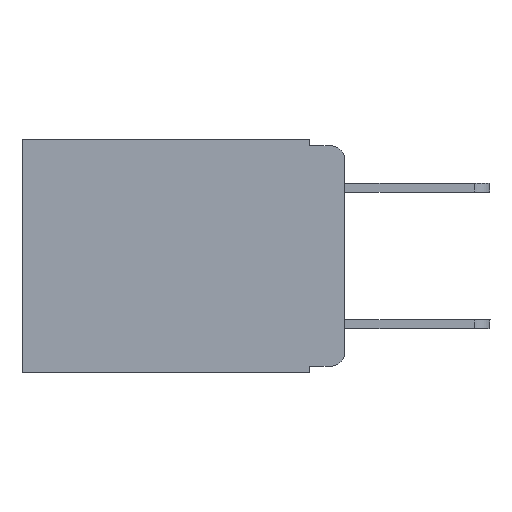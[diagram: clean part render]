
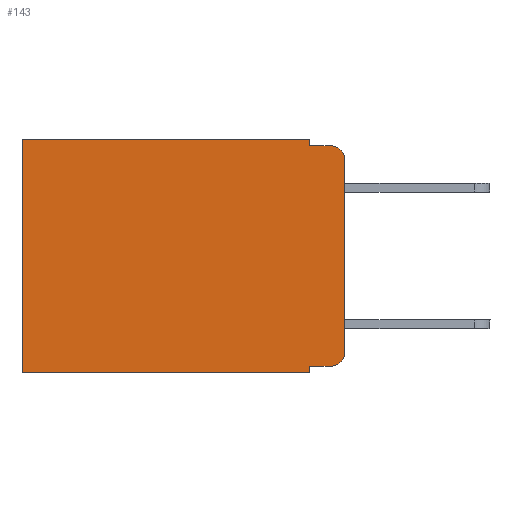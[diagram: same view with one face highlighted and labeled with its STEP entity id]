
A CAD part, left-side view. The second image highlights one B-rep face of the part: STEP entity #143.
In plain terms, the highlighted planar face has unit normal (-1, 0, 0).
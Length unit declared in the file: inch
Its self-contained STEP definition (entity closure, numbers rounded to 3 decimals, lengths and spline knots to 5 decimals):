
#33 = VERTEX_POINT ( 'NONE', #988 ) ;
#143 = ADVANCED_FACE ( 'NONE', ( #11187 ), #699, .F. ) ;
#487 = ORIENTED_EDGE ( 'NONE', *, *, #12742, .T. ) ;
#530 = CARTESIAN_POINT ( 'NONE',  ( 0.298, 0., 0. ) ) ;
#699 = PLANE ( 'NONE',  #9173 ) ;
#811 = CARTESIAN_POINT ( 'NONE',  ( 0.298, 0.02, -0.03 ) ) ;
#978 = LINE ( 'NONE', #1427, #16154 ) ;
#988 = CARTESIAN_POINT ( 'NONE',  ( 0.298, 0., -0.03 ) ) ;
#1113 = LINE ( 'NONE', #8055, #15606 ) ;
#1183 = LINE ( 'NONE', #4387, #14822 ) ;
#1300 = CARTESIAN_POINT ( 'NONE',  ( 0.298, 0., -0.343 ) ) ;
#1375 = EDGE_CURVE ( 'NONE', #7116, #10123, #978, .T. ) ;
#1427 = CARTESIAN_POINT ( 'NONE',  ( 0.298, 0.473, 0. ) ) ;
#1763 = LINE ( 'NONE', #530, #5654 ) ;
#1781 = EDGE_CURVE ( 'NONE', #33, #12541, #6381, .T. ) ;
#1877 = CARTESIAN_POINT ( 'NONE',  ( 0.298, 0., -0.313 ) ) ;
#1934 = CARTESIAN_POINT ( 'NONE',  ( 0.298, 0.051, 0. ) ) ;
#2156 = DIRECTION ( 'NONE',  ( 0., 0., -1. ) ) ;
#2339 = CARTESIAN_POINT ( 'NONE',  ( 0.298, 0.051, -0.333 ) ) ;
#2391 = DIRECTION ( 'NONE',  ( -1., 0., 0. ) ) ;
#2654 = VECTOR ( 'NONE', #15535, 39.37008 ) ;
#2884 = LINE ( 'NONE', #7291, #2654 ) ;
#3006 = CARTESIAN_POINT ( 'NONE',  ( 0.298, 0.02, -0.01 ) ) ;
#3070 = CARTESIAN_POINT ( 'NONE',  ( 0.298, 0.473, 0. ) ) ;
#3205 = LINE ( 'NONE', #7693, #15541 ) ;
#3398 = DIRECTION ( 'NONE',  ( -1., 0., 0. ) ) ;
#3602 = CIRCLE ( 'NONE', #17413, 0.02 ) ;
#3733 = EDGE_CURVE ( 'NONE', #12563, #12300, #2884, .T. ) ;
#3785 = CARTESIAN_POINT ( 'NONE',  ( 0.298, 0.02, -0.333 ) ) ;
#4387 = CARTESIAN_POINT ( 'NONE',  ( 0.298, 0.051, -0.333 ) ) ;
#4423 = EDGE_LOOP ( 'NONE', ( #15699, #9035, #10296, #15743, #487, #11450, #8967, #17879, #5829, #17066 ) ) ;
#4479 = EDGE_CURVE ( 'NONE', #12300, #10123, #14312, .T. ) ;
#4871 = CARTESIAN_POINT ( 'NONE',  ( 0.298, 0., 0. ) ) ;
#5654 = VECTOR ( 'NONE', #8736, 39.37008 ) ;
#5659 = CARTESIAN_POINT ( 'NONE',  ( 0.298, 0.051, -0.01 ) ) ;
#5804 = VERTEX_POINT ( 'NONE', #16118 ) ;
#5829 = ORIENTED_EDGE ( 'NONE', *, *, #7217, .T. ) ;
#6247 = DIRECTION ( 'NONE',  ( 1., 0., 0. ) ) ;
#6308 = VECTOR ( 'NONE', #10950, 39.37008 ) ;
#6381 = CIRCLE ( 'NONE', #12147, 0.02 ) ;
#6781 = VERTEX_POINT ( 'NONE', #1877 ) ;
#7116 = VERTEX_POINT ( 'NONE', #3070 ) ;
#7217 = EDGE_CURVE ( 'NONE', #12563, #13384, #1183, .T. ) ;
#7291 = CARTESIAN_POINT ( 'NONE',  ( 0.298, 0.051, 0. ) ) ;
#7483 = DIRECTION ( 'NONE',  ( 0., 0., -1. ) ) ;
#7693 = CARTESIAN_POINT ( 'NONE',  ( 0.298, 0., 0. ) ) ;
#8055 = CARTESIAN_POINT ( 'NONE',  ( 0.298, 0.051, 0. ) ) ;
#8473 = DIRECTION ( 'NONE',  ( 0., -1., 0. ) ) ;
#8688 = CARTESIAN_POINT ( 'NONE',  ( 0.298, 0.02, -0.313 ) ) ;
#8736 = DIRECTION ( 'NONE',  ( 0., 1., 0. ) ) ;
#8967 = ORIENTED_EDGE ( 'NONE', *, *, #4479, .F. ) ;
#9035 = ORIENTED_EDGE ( 'NONE', *, *, #1781, .T. ) ;
#9173 = AXIS2_PLACEMENT_3D ( 'NONE', #4871, #6247, #11904 ) ;
#9811 = CARTESIAN_POINT ( 'NONE',  ( 0.298, 0.473, -0.343 ) ) ;
#10123 = VERTEX_POINT ( 'NONE', #9811 ) ;
#10296 = ORIENTED_EDGE ( 'NONE', *, *, #13130, .F. ) ;
#10950 = DIRECTION ( 'NONE',  ( 0., 1., 0. ) ) ;
#10957 = DIRECTION ( 'NONE',  ( 0., 0., -1. ) ) ;
#11021 = LINE ( 'NONE', #5659, #13626 ) ;
#11187 = FACE_OUTER_BOUND ( 'NONE', #4423, .T. ) ;
#11450 = ORIENTED_EDGE ( 'NONE', *, *, #1375, .T. ) ;
#11904 = DIRECTION ( 'NONE',  ( 0., 0., -1. ) ) ;
#12043 = DIRECTION ( 'NONE',  ( 0., 0., -1. ) ) ;
#12071 = EDGE_CURVE ( 'NONE', #13384, #6781, #3602, .T. ) ;
#12147 = AXIS2_PLACEMENT_3D ( 'NONE', #811, #2391, #2156 ) ;
#12300 = VERTEX_POINT ( 'NONE', #13582 ) ;
#12541 = VERTEX_POINT ( 'NONE', #3006 ) ;
#12563 = VERTEX_POINT ( 'NONE', #2339 ) ;
#12694 = VERTEX_POINT ( 'NONE', #1934 ) ;
#12742 = EDGE_CURVE ( 'NONE', #12694, #7116, #1763, .T. ) ;
#12939 = EDGE_CURVE ( 'NONE', #12694, #5804, #1113, .T. ) ;
#13130 = EDGE_CURVE ( 'NONE', #5804, #12541, #11021, .T. ) ;
#13384 = VERTEX_POINT ( 'NONE', #3785 ) ;
#13582 = CARTESIAN_POINT ( 'NONE',  ( 0.298, 0.051, -0.343 ) ) ;
#13626 = VECTOR ( 'NONE', #13753, 39.37008 ) ;
#13633 = DIRECTION ( 'NONE',  ( 0., 0., -1. ) ) ;
#13753 = DIRECTION ( 'NONE',  ( 0., -1., 0. ) ) ;
#14312 = LINE ( 'NONE', #1300, #6308 ) ;
#14822 = VECTOR ( 'NONE', #8473, 39.37008 ) ;
#15535 = DIRECTION ( 'NONE',  ( 0., 0., -1. ) ) ;
#15541 = VECTOR ( 'NONE', #12043, 39.37008 ) ;
#15606 = VECTOR ( 'NONE', #13633, 39.37008 ) ;
#15699 = ORIENTED_EDGE ( 'NONE', *, *, #15772, .F. ) ;
#15743 = ORIENTED_EDGE ( 'NONE', *, *, #12939, .F. ) ;
#15772 = EDGE_CURVE ( 'NONE', #33, #6781, #3205, .T. ) ;
#16118 = CARTESIAN_POINT ( 'NONE',  ( 0.298, 0.051, -0.01 ) ) ;
#16154 = VECTOR ( 'NONE', #10957, 39.37008 ) ;
#17066 = ORIENTED_EDGE ( 'NONE', *, *, #12071, .T. ) ;
#17413 = AXIS2_PLACEMENT_3D ( 'NONE', #8688, #3398, #7483 ) ;
#17879 = ORIENTED_EDGE ( 'NONE', *, *, #3733, .F. ) ;
